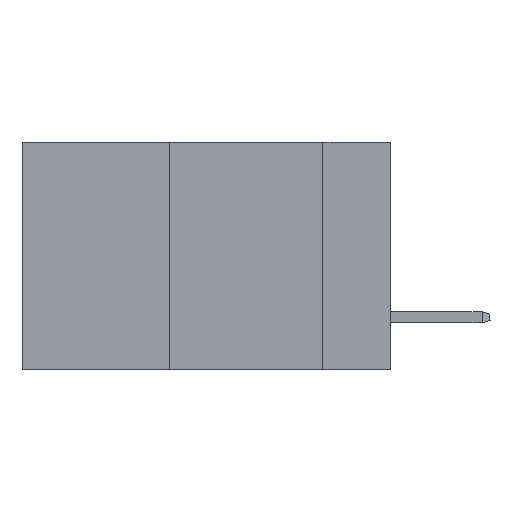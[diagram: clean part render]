
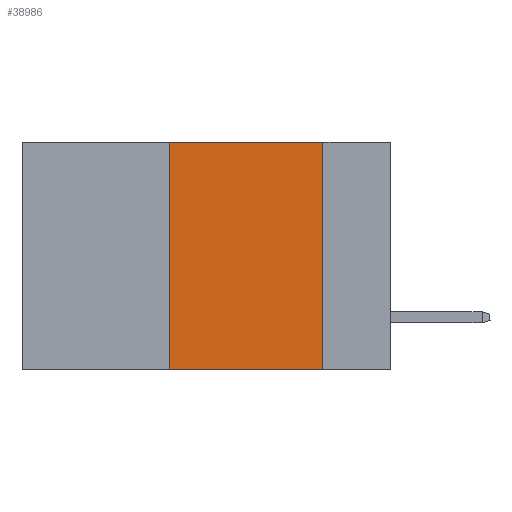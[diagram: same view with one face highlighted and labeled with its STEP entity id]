
A CAD part, left-side view. The second image highlights one B-rep face of the part: STEP entity #38986.
In plain terms, the highlighted planar face has unit normal (-1, 0, 0).
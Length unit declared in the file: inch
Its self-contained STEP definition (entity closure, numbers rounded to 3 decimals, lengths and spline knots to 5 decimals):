
#651 = EDGE_CURVE ( 'NONE', #28095, #10179, #5946, .T. ) ;
#1216 = VECTOR ( 'NONE', #27276, 39.37008 ) ;
#1664 = AXIS2_PLACEMENT_3D ( 'NONE', #25126, #15815, #6105 ) ;
#1946 = CARTESIAN_POINT ( 'NONE',  ( 0., 0.11, -0.37 ) ) ;
#2389 = DIRECTION ( 'NONE',  ( 0., -1., 0. ) ) ;
#3164 = EDGE_CURVE ( 'NONE', #10179, #11502, #27095, .T. ) ;
#4183 = CARTESIAN_POINT ( 'NONE',  ( 0., 0.6, 0. ) ) ;
#5404 = CARTESIAN_POINT ( 'NONE',  ( 0., 0.11, 0. ) ) ;
#5946 = LINE ( 'NONE', #4183, #13884 ) ;
#6105 = DIRECTION ( 'NONE',  ( 0., 0., -1. ) ) ;
#6938 = DIRECTION ( 'NONE',  ( 0., 0., 1. ) ) ;
#7325 = EDGE_CURVE ( 'NONE', #8930, #28095, #15550, .T. ) ;
#7859 = DIRECTION ( 'NONE',  ( 0., 0., -1. ) ) ;
#8366 = ORIENTED_EDGE ( 'NONE', *, *, #13856, .T. ) ;
#8602 = ORIENTED_EDGE ( 'NONE', *, *, #651, .F. ) ;
#8930 = VERTEX_POINT ( 'NONE', #31043 ) ;
#9908 = CARTESIAN_POINT ( 'NONE',  ( 0., 0.36, 0. ) ) ;
#10179 = VERTEX_POINT ( 'NONE', #5404 ) ;
#11033 = FACE_OUTER_BOUND ( 'NONE', #40414, .T. ) ;
#11502 = VERTEX_POINT ( 'NONE', #1946 ) ;
#12674 = CARTESIAN_POINT ( 'NONE',  ( 0., 0.36, 0. ) ) ;
#13856 = EDGE_CURVE ( 'NONE', #8930, #11502, #18150, .T. ) ;
#13884 = VECTOR ( 'NONE', #2389, 39.37008 ) ;
#15550 = LINE ( 'NONE', #12674, #29879 ) ;
#15815 = DIRECTION ( 'NONE',  ( 1., 0., 0. ) ) ;
#18150 = LINE ( 'NONE', #24252, #1216 ) ;
#22337 = PLANE ( 'NONE',  #1664 ) ;
#24252 = CARTESIAN_POINT ( 'NONE',  ( 0., 0.6, -0.37 ) ) ;
#25126 = CARTESIAN_POINT ( 'NONE',  ( 0., 0.6, 0. ) ) ;
#25431 = ORIENTED_EDGE ( 'NONE', *, *, #7325, .F. ) ;
#27095 = LINE ( 'NONE', #33161, #35871 ) ;
#27276 = DIRECTION ( 'NONE',  ( 0., -1., 0. ) ) ;
#28095 = VERTEX_POINT ( 'NONE', #9908 ) ;
#29879 = VECTOR ( 'NONE', #6938, 39.37008 ) ;
#31043 = CARTESIAN_POINT ( 'NONE',  ( 0., 0.36, -0.37 ) ) ;
#33161 = CARTESIAN_POINT ( 'NONE',  ( 0., 0.11, 0. ) ) ;
#35871 = VECTOR ( 'NONE', #7859, 39.37008 ) ;
#38986 = ADVANCED_FACE ( 'NONE', ( #11033 ), #22337, .F. ) ;
#40094 = ORIENTED_EDGE ( 'NONE', *, *, #3164, .F. ) ;
#40414 = EDGE_LOOP ( 'NONE', ( #40094, #8602, #25431, #8366 ) ) ;
